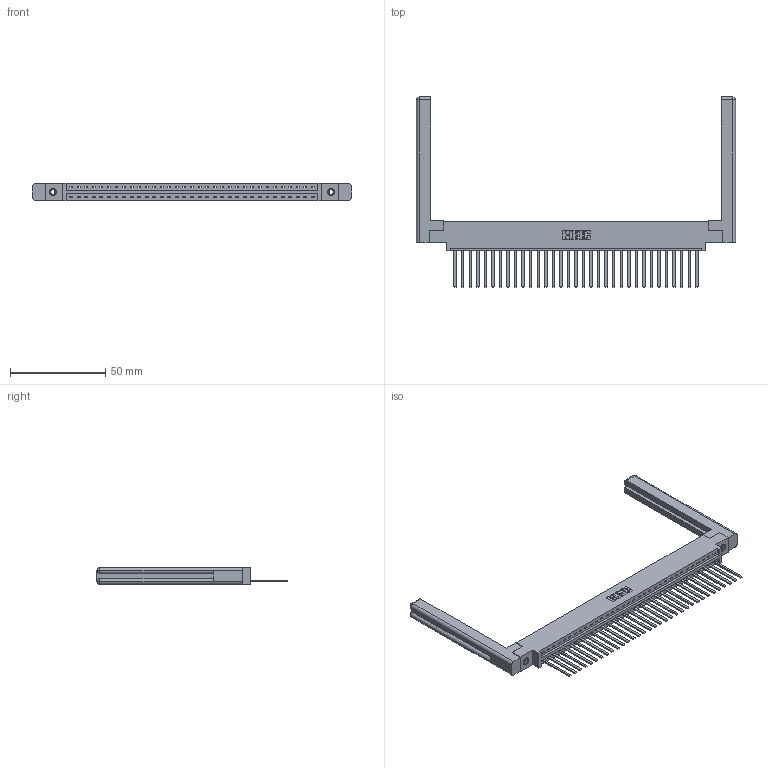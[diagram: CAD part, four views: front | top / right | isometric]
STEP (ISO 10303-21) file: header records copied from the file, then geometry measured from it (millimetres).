
FILE_DESCRIPTION (( 'STEP AP203' ), '1' );
FILE_NAME ('387-033-544-658.STEP', '2019-10-03T22:38:00', ( '' ), ( '' ), 'SwSTEP 2.0', 'SolidWorks 2016', '' );
FILE_SCHEMA (( 'CONFIG_CONTROL_DESIGN' ));
Length unit declared in the file: inch
Products named in the file (5): 345-292-001_345-293-144; 307-220-058; 387-033-544-658; 345-250-001_345-250-001-102; 337 Part_0.170 Offset - 0.156 Dia-TI
Assembly tree (38 placements, depth 2):
  387-033-544-658
    337 Part_0.170 Offset - 0.156 Dia-TI
    345-292-001_345-293-144  x33
    345-250-001_345-250-001-102  x2
    307-220-058  x2
Bounding box: 167.39 x 99.7 x 9.4 mm (x, y, z)
Volume: 24711.2 mm3; surface area: 24651 mm2
Topology: 38 solids, 38 shells, 2108 faces, 6287 edges, 4134 vertices
Faces by surface type: plane 1544, cylinder 540, cone 12, torus 12
Entity records: 28276 total; most frequent: CARTESIAN_POINT 4924, ORIENTED_EDGE 4832, DIRECTION 4178, EDGE_CURVE 2416, LINE 2244, VECTOR 2244, VERTEX_POINT 1602, AXIS2_PLACEMENT_3D 967
